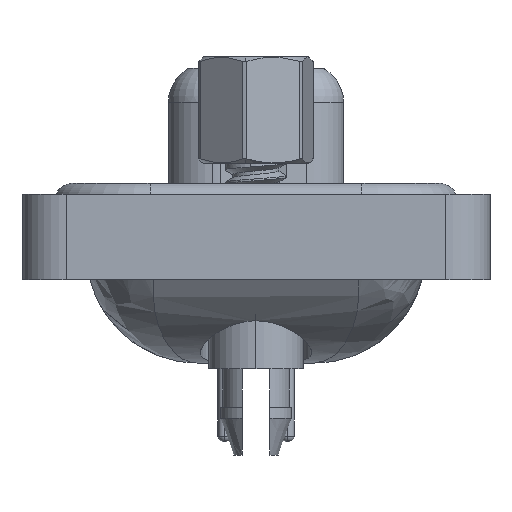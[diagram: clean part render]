
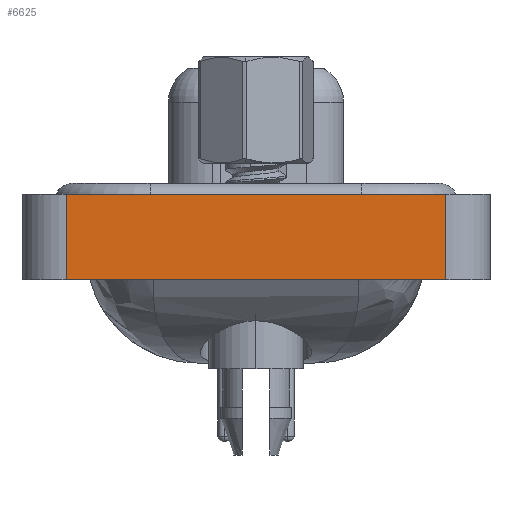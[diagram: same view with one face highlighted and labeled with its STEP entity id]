
A CAD part, left-side view. The second image highlights one B-rep face of the part: STEP entity #6625.
In plain terms, the highlighted planar face has unit normal (-1, 0, 0).
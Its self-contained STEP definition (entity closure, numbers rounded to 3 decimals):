
#57 = DIRECTION ( 'NONE',  ( 0., -1., 0. ) ) ;
#179 = LINE ( 'NONE', #27337, #14095 ) ;
#1801 = LINE ( 'NONE', #15719, #23962 ) ;
#2727 = LINE ( 'NONE', #7897, #25038 ) ;
#3165 = VERTEX_POINT ( 'NONE', #22188 ) ;
#3193 = EDGE_LOOP ( 'NONE', ( #20275, #30071, #6320, #27219 ) ) ;
#6320 = ORIENTED_EDGE ( 'NONE', *, *, #35104, .F. ) ;
#6625 = ADVANCED_FACE ( 'NONE', ( #26647 ), #10406, .T. ) ;
#7847 = DIRECTION ( 'NONE',  ( 0., 0., 1. ) ) ;
#7897 = CARTESIAN_POINT ( 'NONE',  ( -7.15, -8.55, 0.5 ) ) ;
#8312 = VERTEX_POINT ( 'NONE', #32521 ) ;
#10406 = PLANE ( 'NONE',  #31321 ) ;
#12477 = CARTESIAN_POINT ( 'NONE',  ( -7.15, -8.55, -3.35 ) ) ;
#13093 = CARTESIAN_POINT ( 'NONE',  ( -7.15, -8.55, -3.35 ) ) ;
#14095 = VECTOR ( 'NONE', #7847, 1000. ) ;
#15719 = CARTESIAN_POINT ( 'NONE',  ( -7.15, -8.55, -3.35 ) ) ;
#16426 = EDGE_CURVE ( 'NONE', #16781, #3165, #179, .T. ) ;
#16781 = VERTEX_POINT ( 'NONE', #12477 ) ;
#17044 = CARTESIAN_POINT ( 'NONE',  ( -7.15, 8.55, -3.35 ) ) ;
#17874 = EDGE_CURVE ( 'NONE', #22950, #3165, #2727, .T. ) ;
#18266 = DIRECTION ( 'NONE',  ( 0., 0., 1. ) ) ;
#19012 = EDGE_CURVE ( 'NONE', #8312, #16781, #1801, .T. ) ;
#20275 = ORIENTED_EDGE ( 'NONE', *, *, #16426, .T. ) ;
#21124 = DIRECTION ( 'NONE',  ( -1., 0., 0. ) ) ;
#22188 = CARTESIAN_POINT ( 'NONE',  ( -7.15, -8.55, 0.5 ) ) ;
#22685 = VECTOR ( 'NONE', #30612, 1000. ) ;
#22950 = VERTEX_POINT ( 'NONE', #30845 ) ;
#23962 = VECTOR ( 'NONE', #26595, 1000. ) ;
#25038 = VECTOR ( 'NONE', #57, 1000. ) ;
#25606 = LINE ( 'NONE', #17044, #22685 ) ;
#26595 = DIRECTION ( 'NONE',  ( 0., -1., 0. ) ) ;
#26647 = FACE_OUTER_BOUND ( 'NONE', #3193, .T. ) ;
#27219 = ORIENTED_EDGE ( 'NONE', *, *, #19012, .T. ) ;
#27337 = CARTESIAN_POINT ( 'NONE',  ( -7.15, -8.55, -3.35 ) ) ;
#30071 = ORIENTED_EDGE ( 'NONE', *, *, #17874, .F. ) ;
#30612 = DIRECTION ( 'NONE',  ( 0., 0., 1. ) ) ;
#30845 = CARTESIAN_POINT ( 'NONE',  ( -7.15, 8.55, 0.5 ) ) ;
#31321 = AXIS2_PLACEMENT_3D ( 'NONE', #13093, #21124, #18266 ) ;
#32521 = CARTESIAN_POINT ( 'NONE',  ( -7.15, 8.55, -3.35 ) ) ;
#35104 = EDGE_CURVE ( 'NONE', #8312, #22950, #25606, .T. ) ;
